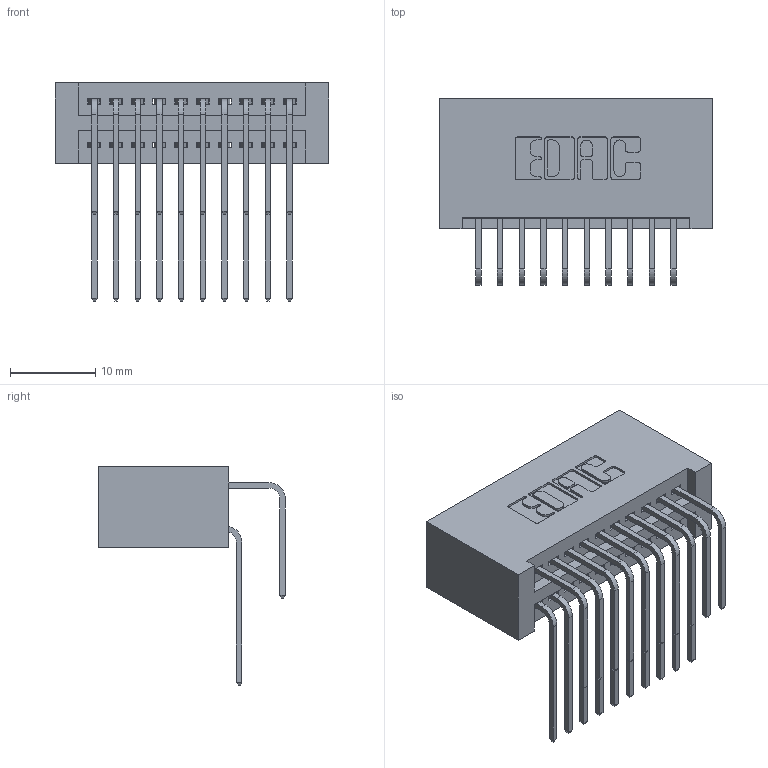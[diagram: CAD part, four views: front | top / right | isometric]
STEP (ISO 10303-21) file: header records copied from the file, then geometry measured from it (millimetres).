
FILE_DESCRIPTION (( 'STEP AP203' ), '1' );
FILE_NAME ('395-020-558-201.STEP', '2018-11-07T19:22:47', ( '' ), ( '' ), 'SwSTEP 2.0', 'SolidWorks 2016', '' );
FILE_SCHEMA (( 'CONFIG_CONTROL_DESIGN' ));
Length unit declared in the file: inch
Products named in the file (4): 345-292-001_558 559 Tail - 1; 345 Part_No Mounting Lugs; 395-020-558-201; 345-292-001_558 Tail - 2
Assembly tree (21 placements, depth 2):
  395-020-558-201
    345 Part_No Mounting Lugs
    345-292-001_558 559 Tail - 1  x10
    345-292-001_558 Tail - 2  x10
Bounding box: 32 x 21.83 x 25.53 mm (x, y, z)
Volume: 3543.1 mm3; surface area: 5463.4 mm2
Topology: 21 solids, 21 shells, 1158 faces, 3417 edges, 2250 vertices
Faces by surface type: plane 776, cylinder 382
Entity records: 13529 total; most frequent: CARTESIAN_POINT 2343, ORIENTED_EDGE 2226, DIRECTION 2073, EDGE_CURVE 1113, VECTOR 909, LINE 909, VERTEX_POINT 738, AXIS2_PLACEMENT_3D 582
